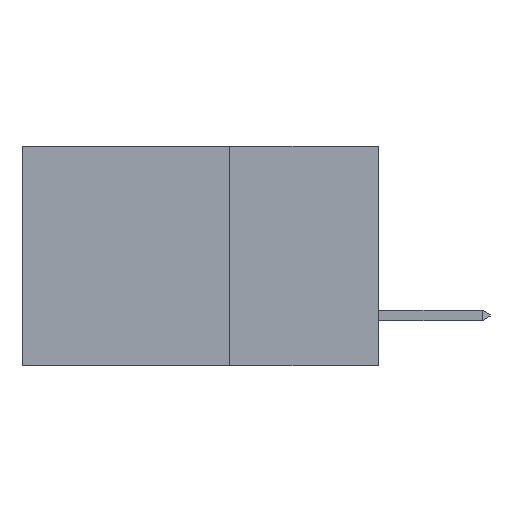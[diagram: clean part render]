
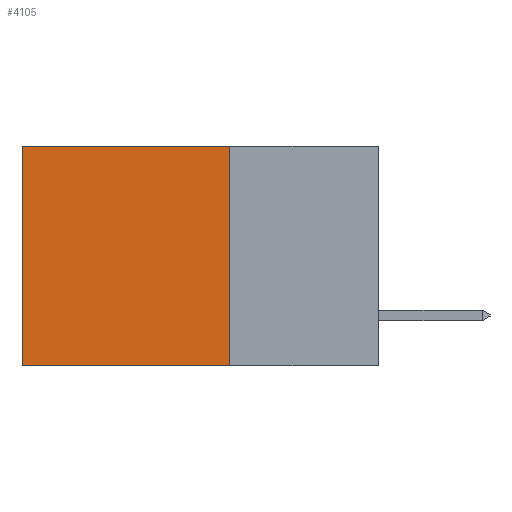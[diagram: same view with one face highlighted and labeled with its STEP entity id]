
A CAD part, left-side view. The second image highlights one B-rep face of the part: STEP entity #4105.
In plain terms, the highlighted planar face has unit normal (-1, 0, 0).
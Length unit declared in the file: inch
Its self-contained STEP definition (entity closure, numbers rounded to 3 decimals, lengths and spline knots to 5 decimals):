
#62 = AXIS2_PLACEMENT_3D ( 'NONE', #722, #6174, #16649 ) ;
#353 = CARTESIAN_POINT ( 'NONE',  ( 0.298, 0.25, 0. ) ) ;
#722 = CARTESIAN_POINT ( 'NONE',  ( 0.298, 0.25, 0. ) ) ;
#942 = EDGE_LOOP ( 'NONE', ( #6532, #12227, #13970, #16259 ) ) ;
#1856 = DIRECTION ( 'NONE',  ( 0., 0., -1. ) ) ;
#1876 = PLANE ( 'NONE',  #62 ) ;
#2378 = VECTOR ( 'NONE', #1856, 39.37008 ) ;
#4105 = ADVANCED_FACE ( 'NONE', ( #7183 ), #1876, .F. ) ;
#6174 = DIRECTION ( 'NONE',  ( 1., 0., 0. ) ) ;
#6218 = LINE ( 'NONE', #353, #2378 ) ;
#6532 = ORIENTED_EDGE ( 'NONE', *, *, #14747, .T. ) ;
#6569 = VECTOR ( 'NONE', #10630, 39.37008 ) ;
#7183 = FACE_OUTER_BOUND ( 'NONE', #942, .T. ) ;
#7487 = LINE ( 'NONE', #13024, #11231 ) ;
#9252 = LINE ( 'NONE', #12255, #12790 ) ;
#10409 = CARTESIAN_POINT ( 'NONE',  ( 0.298, 0.25, -0.37 ) ) ;
#10630 = DIRECTION ( 'NONE',  ( 0., 0., -1. ) ) ;
#10761 = LINE ( 'NONE', #17602, #6569 ) ;
#11023 = CARTESIAN_POINT ( 'NONE',  ( 0.298, 0.6, 0. ) ) ;
#11231 = VECTOR ( 'NONE', #14433, 39.37008 ) ;
#11581 = EDGE_CURVE ( 'NONE', #17789, #14003, #6218, .T. ) ;
#12227 = ORIENTED_EDGE ( 'NONE', *, *, #13550, .F. ) ;
#12255 = CARTESIAN_POINT ( 'NONE',  ( 0.298, 0.25, -0.37 ) ) ;
#12790 = VECTOR ( 'NONE', #13691, 39.37008 ) ;
#13024 = CARTESIAN_POINT ( 'NONE',  ( 0.298, 0.25, 0. ) ) ;
#13244 = EDGE_CURVE ( 'NONE', #17789, #17756, #7487, .T. ) ;
#13550 = EDGE_CURVE ( 'NONE', #14003, #15241, #9252, .T. ) ;
#13691 = DIRECTION ( 'NONE',  ( 0., 1., 0. ) ) ;
#13970 = ORIENTED_EDGE ( 'NONE', *, *, #11581, .F. ) ;
#14003 = VERTEX_POINT ( 'NONE', #10409 ) ;
#14433 = DIRECTION ( 'NONE',  ( 0., 1., 0. ) ) ;
#14542 = CARTESIAN_POINT ( 'NONE',  ( 0.298, 0.6, -0.37 ) ) ;
#14747 = EDGE_CURVE ( 'NONE', #17756, #15241, #10761, .T. ) ;
#15241 = VERTEX_POINT ( 'NONE', #14542 ) ;
#16259 = ORIENTED_EDGE ( 'NONE', *, *, #13244, .T. ) ;
#16649 = DIRECTION ( 'NONE',  ( 0., 0., -1. ) ) ;
#17602 = CARTESIAN_POINT ( 'NONE',  ( 0.298, 0.6, 0. ) ) ;
#17756 = VERTEX_POINT ( 'NONE', #11023 ) ;
#17789 = VERTEX_POINT ( 'NONE', #18048 ) ;
#18048 = CARTESIAN_POINT ( 'NONE',  ( 0.298, 0.25, 0. ) ) ;
